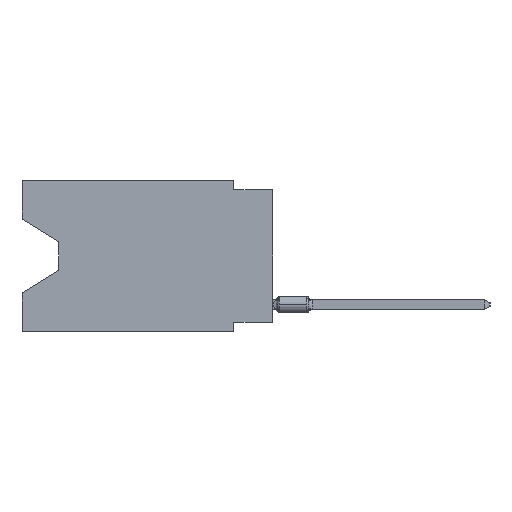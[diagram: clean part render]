
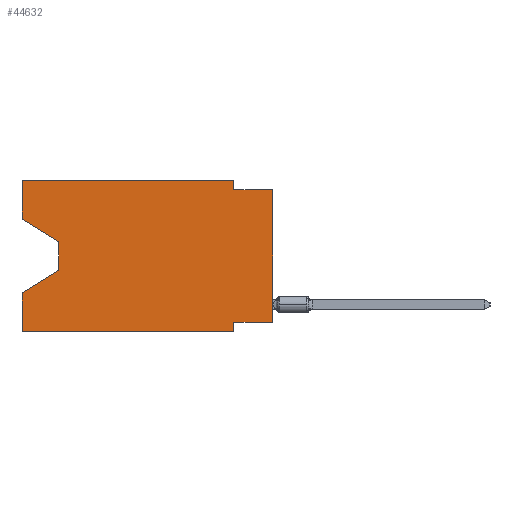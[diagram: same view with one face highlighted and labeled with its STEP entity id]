
A CAD part, left-side view. The second image highlights one B-rep face of the part: STEP entity #44632.
In plain terms, the highlighted planar face has unit normal (-1, 0, 0).
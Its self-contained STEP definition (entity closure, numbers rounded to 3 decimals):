
#389 = CARTESIAN_POINT ( 'NONE',  ( 0., 0., 0. ) ) ;
#1239 = EDGE_CURVE ( 'NONE', #49733, #34477, #25225, .T. ) ;
#2487 = EDGE_CURVE ( 'NONE', #49733, #7015, #41598, .T. ) ;
#2967 = ORIENTED_EDGE ( 'NONE', *, *, #3466, .F. ) ;
#3466 = EDGE_CURVE ( 'NONE', #7015, #15057, #36090, .T. ) ;
#3554 = LINE ( 'NONE', #50630, #34183 ) ;
#4302 = DIRECTION ( 'NONE',  ( 0., -1., 0. ) ) ;
#5139 = VERTEX_POINT ( 'NONE', #39459 ) ;
#5291 = DIRECTION ( 'NONE',  ( 0., 0., -1. ) ) ;
#5339 = VERTEX_POINT ( 'NONE', #16920 ) ;
#5569 = ORIENTED_EDGE ( 'NONE', *, *, #21914, .T. ) ;
#6074 = CARTESIAN_POINT ( 'NONE',  ( 0., 2.54, 0. ) ) ;
#6602 = CARTESIAN_POINT ( 'NONE',  ( 0., 2.54, -9.906 ) ) ;
#7015 = VERTEX_POINT ( 'NONE', #24187 ) ;
#7135 = VERTEX_POINT ( 'NONE', #29336 ) ;
#7291 = CARTESIAN_POINT ( 'NONE',  ( 0., 16.383, 0. ) ) ;
#8064 = VECTOR ( 'NONE', #44102, 1000. ) ;
#8364 = DIRECTION ( 'NONE',  ( 0., 0., 1. ) ) ;
#8543 = CARTESIAN_POINT ( 'NONE',  ( 0., 16.383, 0. ) ) ;
#8880 = VECTOR ( 'NONE', #46094, 1000. ) ;
#9972 = VECTOR ( 'NONE', #5291, 1000. ) ;
#10391 = CARTESIAN_POINT ( 'NONE',  ( 0., 0., -0.635 ) ) ;
#10609 = EDGE_CURVE ( 'NONE', #5139, #5339, #30038, .T. ) ;
#11217 = DIRECTION ( 'NONE',  ( 0., 0., -1. ) ) ;
#11949 = VECTOR ( 'NONE', #13428, 1000. ) ;
#12323 = ORIENTED_EDGE ( 'NONE', *, *, #47818, .F. ) ;
#13312 = CARTESIAN_POINT ( 'NONE',  ( 0., 13.97, -4.013 ) ) ;
#13428 = DIRECTION ( 'NONE',  ( 0., 0., 1. ) ) ;
#13687 = LINE ( 'NONE', #8543, #11949 ) ;
#14295 = DIRECTION ( 'NONE',  ( 1., 0., 0. ) ) ;
#14742 = CARTESIAN_POINT ( 'NONE',  ( 0., 0., -9.271 ) ) ;
#15057 = VERTEX_POINT ( 'NONE', #6602 ) ;
#15501 = EDGE_CURVE ( 'NONE', #41317, #32072, #34735, .T. ) ;
#16466 = VERTEX_POINT ( 'NONE', #13312 ) ;
#16920 = CARTESIAN_POINT ( 'NONE',  ( 0., 16.383, -7.36 ) ) ;
#17666 = LINE ( 'NONE', #29312, #35022 ) ;
#17803 = VERTEX_POINT ( 'NONE', #18773 ) ;
#17866 = ORIENTED_EDGE ( 'NONE', *, *, #42079, .F. ) ;
#18621 = EDGE_CURVE ( 'NONE', #7135, #5339, #48171, .T. ) ;
#18773 = CARTESIAN_POINT ( 'NONE',  ( 0., 16.383, 0. ) ) ;
#18942 = DIRECTION ( 'NONE',  ( 0., -1., 0. ) ) ;
#19815 = CARTESIAN_POINT ( 'NONE',  ( 0., 0., -0.635 ) ) ;
#20912 = CARTESIAN_POINT ( 'NONE',  ( 0., 0., -9.271 ) ) ;
#21328 = CARTESIAN_POINT ( 'NONE',  ( 0., 2.54, -9.906 ) ) ;
#21369 = VECTOR ( 'NONE', #25550, 1000. ) ;
#21548 = EDGE_CURVE ( 'NONE', #32072, #34477, #26181, .T. ) ;
#21914 = EDGE_CURVE ( 'NONE', #16466, #5139, #26495, .T. ) ;
#22019 = ORIENTED_EDGE ( 'NONE', *, *, #21548, .F. ) ;
#23463 = EDGE_CURVE ( 'NONE', #50165, #16466, #17666, .T. ) ;
#23784 = VECTOR ( 'NONE', #8364, 1000. ) ;
#24187 = CARTESIAN_POINT ( 'NONE',  ( 0., 2.54, -9.271 ) ) ;
#25225 = LINE ( 'NONE', #389, #8064 ) ;
#25508 = ORIENTED_EDGE ( 'NONE', *, *, #23463, .T. ) ;
#25550 = DIRECTION ( 'NONE',  ( 0., 1., 0. ) ) ;
#25932 = DIRECTION ( 'NONE',  ( 0., -1., 0. ) ) ;
#25946 = CARTESIAN_POINT ( 'NONE',  ( 0., 16.383, 0. ) ) ;
#26151 = DIRECTION ( 'NONE',  ( 0., 0.855, -0.519 ) ) ;
#26181 = LINE ( 'NONE', #10391, #34867 ) ;
#26495 = LINE ( 'NONE', #31158, #44766 ) ;
#28532 = CARTESIAN_POINT ( 'NONE',  ( 0., 16.383, 0. ) ) ;
#28560 = ORIENTED_EDGE ( 'NONE', *, *, #1239, .T. ) ;
#29312 = CARTESIAN_POINT ( 'NONE',  ( 0., 16.383, -2.546 ) ) ;
#29336 = CARTESIAN_POINT ( 'NONE',  ( 0., 16.383, -9.906 ) ) ;
#29993 = ORIENTED_EDGE ( 'NONE', *, *, #2487, .F. ) ;
#30038 = LINE ( 'NONE', #45795, #34973 ) ;
#30867 = CARTESIAN_POINT ( 'NONE',  ( 0., 2.54, 0. ) ) ;
#31158 = CARTESIAN_POINT ( 'NONE',  ( 0., 13.97, -4.013 ) ) ;
#31227 = AXIS2_PLACEMENT_3D ( 'NONE', #25946, #14295, #45328 ) ;
#31684 = ORIENTED_EDGE ( 'NONE', *, *, #10609, .T. ) ;
#32072 = VERTEX_POINT ( 'NONE', #33845 ) ;
#32213 = EDGE_CURVE ( 'NONE', #7135, #15057, #3554, .T. ) ;
#32551 = ORIENTED_EDGE ( 'NONE', *, *, #18621, .F. ) ;
#33845 = CARTESIAN_POINT ( 'NONE',  ( 0., 2.54, -0.635 ) ) ;
#34183 = VECTOR ( 'NONE', #4302, 1000. ) ;
#34477 = VERTEX_POINT ( 'NONE', #19815 ) ;
#34735 = LINE ( 'NONE', #30867, #8880 ) ;
#34867 = VECTOR ( 'NONE', #25932, 1000. ) ;
#34973 = VECTOR ( 'NONE', #26151, 1000. ) ;
#35022 = VECTOR ( 'NONE', #44813, 1000. ) ;
#36090 = LINE ( 'NONE', #21328, #9972 ) ;
#37350 = PLANE ( 'NONE',  #31227 ) ;
#37601 = FACE_OUTER_BOUND ( 'NONE', #38427, .T. ) ;
#37746 = CARTESIAN_POINT ( 'NONE',  ( 0., 16.383, -2.546 ) ) ;
#38427 = EDGE_LOOP ( 'NONE', ( #25508, #5569, #31684, #32551, #44364, #2967, #29993, #28560, #22019, #48163, #12323, #17866 ) ) ;
#39459 = CARTESIAN_POINT ( 'NONE',  ( 0., 13.97, -5.893 ) ) ;
#41317 = VERTEX_POINT ( 'NONE', #6074 ) ;
#41598 = LINE ( 'NONE', #20912, #21369 ) ;
#42079 = EDGE_CURVE ( 'NONE', #50165, #17803, #13687, .T. ) ;
#44102 = DIRECTION ( 'NONE',  ( 0., 0., 1. ) ) ;
#44364 = ORIENTED_EDGE ( 'NONE', *, *, #32213, .T. ) ;
#44632 = ADVANCED_FACE ( 'NONE', ( #37601 ), #37350, .F. ) ;
#44766 = VECTOR ( 'NONE', #11217, 1000. ) ;
#44813 = DIRECTION ( 'NONE',  ( 0., -0.855, -0.519 ) ) ;
#45328 = DIRECTION ( 'NONE',  ( 0., 0., -1. ) ) ;
#45795 = CARTESIAN_POINT ( 'NONE',  ( 0., 13.97, -5.893 ) ) ;
#46094 = DIRECTION ( 'NONE',  ( 0., 0., -1. ) ) ;
#47818 = EDGE_CURVE ( 'NONE', #17803, #41317, #49455, .T. ) ;
#48163 = ORIENTED_EDGE ( 'NONE', *, *, #15501, .F. ) ;
#48171 = LINE ( 'NONE', #28532, #23784 ) ;
#49455 = LINE ( 'NONE', #7291, #51153 ) ;
#49733 = VERTEX_POINT ( 'NONE', #14742 ) ;
#50165 = VERTEX_POINT ( 'NONE', #37746 ) ;
#50630 = CARTESIAN_POINT ( 'NONE',  ( 0., 16.383, -9.906 ) ) ;
#51153 = VECTOR ( 'NONE', #18942, 1000. ) ;
